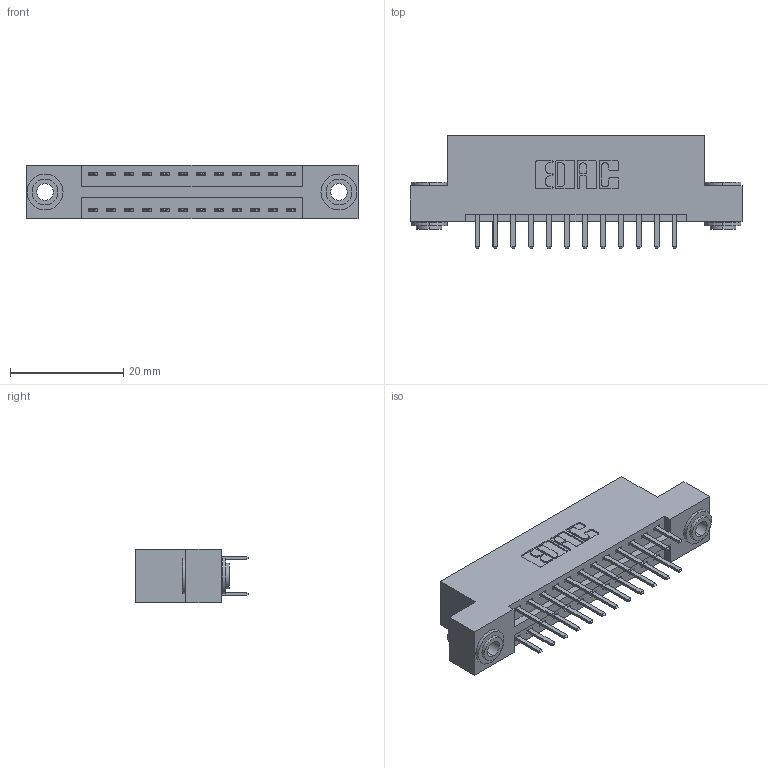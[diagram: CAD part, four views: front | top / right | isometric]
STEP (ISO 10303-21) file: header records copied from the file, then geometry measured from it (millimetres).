
FILE_DESCRIPTION (( 'STEP AP203' ), '1' );
FILE_NAME ('396-024-520-203.STEP', '2019-10-30T04:03:11', ( '' ), ( '' ), 'SwSTEP 2.0', 'SolidWorks 2016', '' );
FILE_SCHEMA (( 'CONFIG_CONTROL_DESIGN' ));
Length unit declared in the file: inch
Products named in the file (4): 396-024-520-203; 345-292-001_345-293-120; 345-250-002_345-250-002-102; 346 Part_Flush Mounting Lugs - 0.156 Dia-TH
Assembly tree (27 placements, depth 2):
  396-024-520-203
    346 Part_Flush Mounting Lugs - 0.156 Dia-TH
    345-292-001_345-293-120  x24
    345-250-002_345-250-002-102  x2
Bounding box: 58.67 x 20.02 x 9.4 mm (x, y, z)
Volume: 5497.3 mm3; surface area: 7274.3 mm2
Topology: 27 solids, 27 shells, 1504 faces, 4317 edges, 2810 vertices
Faces by surface type: plane 974, cylinder 522, cone 8
Entity records: 12634 total; most frequent: CARTESIAN_POINT 2111, ORIENTED_EDGE 2026, DIRECTION 1931, EDGE_CURVE 1013, LINE 805, VECTOR 805, VERTEX_POINT 670, AXIS2_PLACEMENT_3D 563
